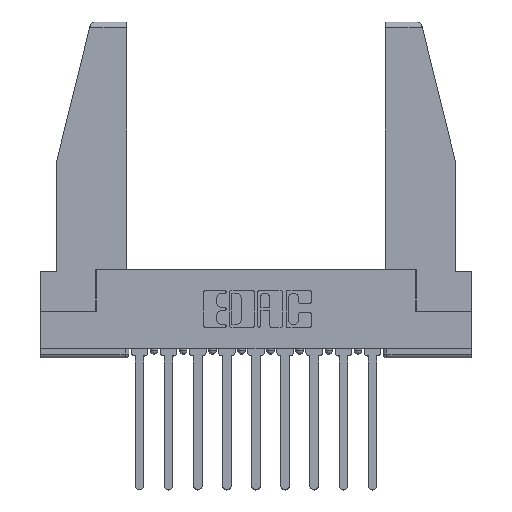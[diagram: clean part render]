
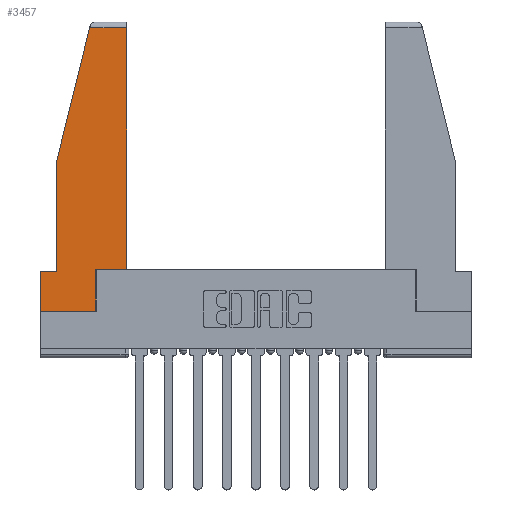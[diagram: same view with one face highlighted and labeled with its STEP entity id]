
A CAD part, top view. The second image highlights one B-rep face of the part: STEP entity #3457.
In plain terms, the highlighted planar face has unit normal (0, 0, 1).
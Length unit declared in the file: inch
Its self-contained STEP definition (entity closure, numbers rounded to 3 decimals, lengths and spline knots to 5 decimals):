
#62 = DIRECTION ( 'NONE',  ( 0., 1., 0. ) ) ;
#560 = CARTESIAN_POINT ( 'NONE',  ( 0.297, 0.223, 0. ) ) ;
#569 = CARTESIAN_POINT ( 'NONE',  ( 0.271, 1.55, 0. ) ) ;
#974 = CARTESIAN_POINT ( 'NONE',  ( 0., 0.21, 0. ) ) ;
#1173 = VECTOR ( 'NONE', #5333, 39.37008 ) ;
#1432 = EDGE_CURVE ( 'NONE', #12739, #9497, #7712, .T. ) ;
#1792 = EDGE_CURVE ( 'NONE', #2167, #5795, #4339, .T. ) ;
#2159 = DIRECTION ( 'NONE',  ( -1., 0., 0. ) ) ;
#2167 = VERTEX_POINT ( 'NONE', #13071 ) ;
#2230 = VECTOR ( 'NONE', #12245, 39.37008 ) ;
#2253 = ORIENTED_EDGE ( 'NONE', *, *, #2310, .T. ) ;
#2297 = CARTESIAN_POINT ( 'NONE',  ( 0.297, 0., 0. ) ) ;
#2310 = EDGE_CURVE ( 'NONE', #9302, #7183, #6653, .T. ) ;
#2387 = LINE ( 'NONE', #560, #8876 ) ;
#2612 = DIRECTION ( 'NONE',  ( 1., 0., 0. ) ) ;
#2832 = LINE ( 'NONE', #12191, #11416 ) ;
#2960 = CARTESIAN_POINT ( 'NONE',  ( 0.297, 0.223, 0. ) ) ;
#3372 = DIRECTION ( 'NONE',  ( 0., 1., 0. ) ) ;
#3457 = ADVANCED_FACE ( 'NONE', ( #4101 ), #6265, .T. ) ;
#3629 = LINE ( 'NONE', #2297, #8393 ) ;
#3720 = CARTESIAN_POINT ( 'NONE',  ( 0.297, 0., 0. ) ) ;
#4080 = DIRECTION ( 'NONE',  ( 0., 0., 1. ) ) ;
#4101 = FACE_OUTER_BOUND ( 'NONE', #9998, .T. ) ;
#4211 = EDGE_CURVE ( 'NONE', #7183, #9308, #3629, .T. ) ;
#4339 = LINE ( 'NONE', #14451, #9088 ) ;
#5141 = LINE ( 'NONE', #10029, #8848 ) ;
#5156 = DIRECTION ( 'NONE',  ( 0., -1., 0. ) ) ;
#5333 = DIRECTION ( 'NONE',  ( 1., 0., 0. ) ) ;
#5586 = ORIENTED_EDGE ( 'NONE', *, *, #1792, .T. ) ;
#5795 = VERTEX_POINT ( 'NONE', #9000 ) ;
#6031 = EDGE_CURVE ( 'NONE', #9308, #2167, #2387, .T. ) ;
#6265 = PLANE ( 'NONE',  #11518 ) ;
#6266 = CARTESIAN_POINT ( 'NONE',  ( 0., 0., 0. ) ) ;
#6474 = CARTESIAN_POINT ( 'NONE',  ( 0.2636, 1.52, 0. ) ) ;
#6632 = CARTESIAN_POINT ( 'NONE',  ( 0.086, 0.21, 0. ) ) ;
#6653 = LINE ( 'NONE', #11015, #1173 ) ;
#6739 = ORIENTED_EDGE ( 'NONE', *, *, #7009, .T. ) ;
#6868 = ORIENTED_EDGE ( 'NONE', *, *, #14392, .T. ) ;
#6951 = LINE ( 'NONE', #569, #11301 ) ;
#7009 = EDGE_CURVE ( 'NONE', #10688, #9302, #5141, .T. ) ;
#7142 = CARTESIAN_POINT ( 'NONE',  ( 0.086, 0.8, 0. ) ) ;
#7183 = VERTEX_POINT ( 'NONE', #3720 ) ;
#7400 = CARTESIAN_POINT ( 'NONE',  ( 0., 0., 0. ) ) ;
#7712 = LINE ( 'NONE', #9429, #8400 ) ;
#7796 = DIRECTION ( 'NONE',  ( 0., -1., 0. ) ) ;
#8113 = ORIENTED_EDGE ( 'NONE', *, *, #6031, .T. ) ;
#8393 = VECTOR ( 'NONE', #3372, 39.37008 ) ;
#8400 = VECTOR ( 'NONE', #5156, 39.37008 ) ;
#8548 = ORIENTED_EDGE ( 'NONE', *, *, #13220, .T. ) ;
#8848 = VECTOR ( 'NONE', #7796, 39.37008 ) ;
#8876 = VECTOR ( 'NONE', #2612, 39.37008 ) ;
#9000 = CARTESIAN_POINT ( 'NONE',  ( 0.461, 1.52, 0. ) ) ;
#9029 = ORIENTED_EDGE ( 'NONE', *, *, #4211, .T. ) ;
#9088 = VECTOR ( 'NONE', #62, 39.37008 ) ;
#9302 = VERTEX_POINT ( 'NONE', #6266 ) ;
#9308 = VERTEX_POINT ( 'NONE', #2960 ) ;
#9429 = CARTESIAN_POINT ( 'NONE',  ( 0.086, 0.8, 0. ) ) ;
#9497 = VERTEX_POINT ( 'NONE', #6632 ) ;
#9998 = EDGE_LOOP ( 'NONE', ( #5586, #8548, #6868, #12499, #12132, #6739, #2253, #9029, #8113 ) ) ;
#10029 = CARTESIAN_POINT ( 'NONE',  ( 0., 0.21, 0. ) ) ;
#10156 = EDGE_CURVE ( 'NONE', #9497, #10688, #2832, .T. ) ;
#10688 = VERTEX_POINT ( 'NONE', #974 ) ;
#11015 = CARTESIAN_POINT ( 'NONE',  ( 0., 0., 0. ) ) ;
#11125 = CARTESIAN_POINT ( 'NONE',  ( 0., 1.52, 0. ) ) ;
#11301 = VECTOR ( 'NONE', #14063, 39.37008 ) ;
#11364 = VERTEX_POINT ( 'NONE', #6474 ) ;
#11416 = VECTOR ( 'NONE', #2159, 39.37008 ) ;
#11448 = DIRECTION ( 'NONE',  ( 1., 0., 0. ) ) ;
#11518 = AXIS2_PLACEMENT_3D ( 'NONE', #7400, #4080, #11448 ) ;
#12132 = ORIENTED_EDGE ( 'NONE', *, *, #10156, .T. ) ;
#12191 = CARTESIAN_POINT ( 'NONE',  ( 0., 0.21, 0. ) ) ;
#12245 = DIRECTION ( 'NONE',  ( -1., 0., 0. ) ) ;
#12499 = ORIENTED_EDGE ( 'NONE', *, *, #1432, .T. ) ;
#12739 = VERTEX_POINT ( 'NONE', #7142 ) ;
#13071 = CARTESIAN_POINT ( 'NONE',  ( 0.461, 0.223, 0. ) ) ;
#13220 = EDGE_CURVE ( 'NONE', #5795, #11364, #14127, .T. ) ;
#14063 = DIRECTION ( 'NONE',  ( -0.239, -0.971, 0. ) ) ;
#14127 = LINE ( 'NONE', #11125, #2230 ) ;
#14392 = EDGE_CURVE ( 'NONE', #11364, #12739, #6951, .T. ) ;
#14451 = CARTESIAN_POINT ( 'NONE',  ( 0.461, 0.223, 0. ) ) ;
